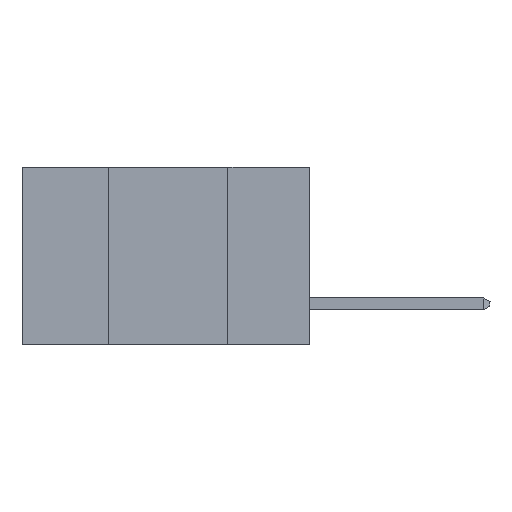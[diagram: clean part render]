
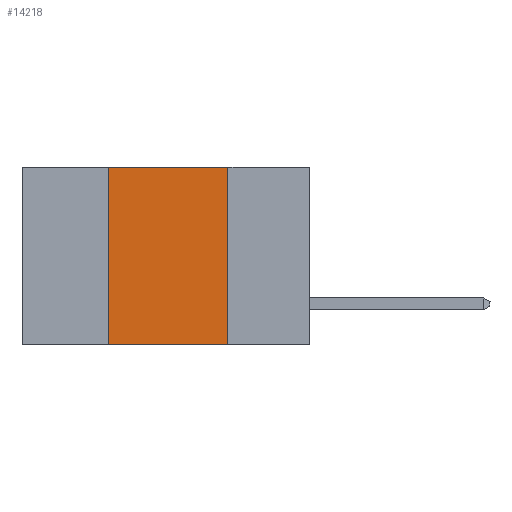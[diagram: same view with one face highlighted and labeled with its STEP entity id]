
A CAD part, left-side view. The second image highlights one B-rep face of the part: STEP entity #14218.
In plain terms, the highlighted planar face has unit normal (-1, 0, 0).
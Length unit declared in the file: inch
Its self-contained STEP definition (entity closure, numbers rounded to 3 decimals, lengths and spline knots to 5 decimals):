
#974 = ORIENTED_EDGE ( 'NONE', *, *, #20174, .T. ) ;
#2215 = EDGE_LOOP ( 'NONE', ( #28649, #23041, #28165, #974 ) ) ;
#2992 = DIRECTION ( 'NONE',  ( 1., 0., 0. ) ) ;
#3809 = LINE ( 'NONE', #20181, #29925 ) ;
#4281 = EDGE_CURVE ( 'NONE', #33150, #14584, #3809, .T. ) ;
#7104 = DIRECTION ( 'NONE',  ( 0., -1., 0. ) ) ;
#9103 = DIRECTION ( 'NONE',  ( 0., 0., -1. ) ) ;
#9169 = CARTESIAN_POINT ( 'NONE',  ( 0., 0.42, -0.37 ) ) ;
#9826 = DIRECTION ( 'NONE',  ( 0., 0., -1. ) ) ;
#10266 = AXIS2_PLACEMENT_3D ( 'NONE', #26670, #2992, #9826 ) ;
#10805 = FACE_OUTER_BOUND ( 'NONE', #2215, .T. ) ;
#11481 = LINE ( 'NONE', #35554, #13058 ) ;
#11754 = VERTEX_POINT ( 'NONE', #20759 ) ;
#11848 = VECTOR ( 'NONE', #9103, 39.37008 ) ;
#13058 = VECTOR ( 'NONE', #43260, 39.37008 ) ;
#13713 = VERTEX_POINT ( 'NONE', #19568 ) ;
#14218 = ADVANCED_FACE ( 'NONE', ( #10805 ), #33654, .F. ) ;
#14584 = VERTEX_POINT ( 'NONE', #31888 ) ;
#14772 = LINE ( 'NONE', #40879, #27560 ) ;
#19344 = EDGE_CURVE ( 'NONE', #14584, #13713, #14772, .T. ) ;
#19568 = CARTESIAN_POINT ( 'NONE',  ( 0., 0.17, 0. ) ) ;
#20174 = EDGE_CURVE ( 'NONE', #33150, #11754, #11481, .T. ) ;
#20181 = CARTESIAN_POINT ( 'NONE',  ( 0., 0.42, 0. ) ) ;
#20759 = CARTESIAN_POINT ( 'NONE',  ( 0., 0.17, -0.37 ) ) ;
#23040 = LINE ( 'NONE', #29976, #11848 ) ;
#23041 = ORIENTED_EDGE ( 'NONE', *, *, #19344, .F. ) ;
#26670 = CARTESIAN_POINT ( 'NONE',  ( 0., 0.6, 0. ) ) ;
#26734 = DIRECTION ( 'NONE',  ( 0., 0., 1. ) ) ;
#27560 = VECTOR ( 'NONE', #7104, 39.37008 ) ;
#28165 = ORIENTED_EDGE ( 'NONE', *, *, #4281, .F. ) ;
#28649 = ORIENTED_EDGE ( 'NONE', *, *, #34321, .F. ) ;
#29925 = VECTOR ( 'NONE', #26734, 39.37008 ) ;
#29976 = CARTESIAN_POINT ( 'NONE',  ( 0., 0.17, 0. ) ) ;
#31888 = CARTESIAN_POINT ( 'NONE',  ( 0., 0.42, 0. ) ) ;
#33150 = VERTEX_POINT ( 'NONE', #9169 ) ;
#33654 = PLANE ( 'NONE',  #10266 ) ;
#34321 = EDGE_CURVE ( 'NONE', #13713, #11754, #23040, .T. ) ;
#35554 = CARTESIAN_POINT ( 'NONE',  ( 0., 0.6, -0.37 ) ) ;
#40879 = CARTESIAN_POINT ( 'NONE',  ( 0., 0.6, 0. ) ) ;
#43260 = DIRECTION ( 'NONE',  ( 0., -1., 0. ) ) ;
